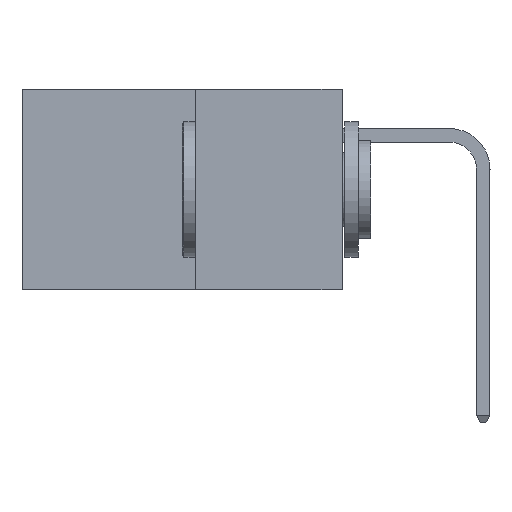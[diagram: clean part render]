
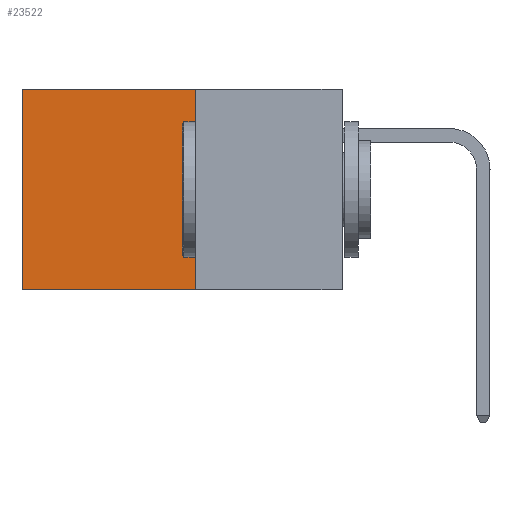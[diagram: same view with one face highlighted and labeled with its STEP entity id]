
A CAD part, left-side view. The second image highlights one B-rep face of the part: STEP entity #23522.
In plain terms, the highlighted planar face has unit normal (-1, 0, 0).
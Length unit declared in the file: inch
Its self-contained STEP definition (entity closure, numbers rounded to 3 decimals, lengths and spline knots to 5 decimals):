
#218 = ORIENTED_EDGE ( 'NONE', *, *, #18377, .T. ) ;
#535 = DIRECTION ( 'NONE',  ( 1., 0., 0. ) ) ;
#880 = LINE ( 'NONE', #8415, #6018 ) ;
#889 = EDGE_LOOP ( 'NONE', ( #14393, #20771, #14347, #218 ) ) ;
#1818 = LINE ( 'NONE', #4591, #18602 ) ;
#1972 = VERTEX_POINT ( 'NONE', #27036 ) ;
#4591 = CARTESIAN_POINT ( 'NONE',  ( 0.277, 0.59, -0.37 ) ) ;
#6018 = VECTOR ( 'NONE', #25820, 39.37008 ) ;
#6804 = DIRECTION ( 'NONE',  ( 0., 0., -1. ) ) ;
#6937 = VECTOR ( 'NONE', #21054, 39.37008 ) ;
#8415 = CARTESIAN_POINT ( 'NONE',  ( 0.277, 0.27, -0.37 ) ) ;
#9565 = DIRECTION ( 'NONE',  ( 0., 1., 0. ) ) ;
#9584 = LINE ( 'NONE', #26789, #14672 ) ;
#11181 = FACE_OUTER_BOUND ( 'NONE', #889, .T. ) ;
#12370 = CARTESIAN_POINT ( 'NONE',  ( 0.277, 0.27, -0.37 ) ) ;
#12713 = LINE ( 'NONE', #12370, #6937 ) ;
#13580 = VERTEX_POINT ( 'NONE', #25212 ) ;
#14347 = ORIENTED_EDGE ( 'NONE', *, *, #17163, .F. ) ;
#14393 = ORIENTED_EDGE ( 'NONE', *, *, #25401, .T. ) ;
#14672 = VECTOR ( 'NONE', #9565, 39.37008 ) ;
#15749 = CARTESIAN_POINT ( 'NONE',  ( 0.277, 0.27, -0.37 ) ) ;
#15768 = CARTESIAN_POINT ( 'NONE',  ( 0.277, 0.59, 0. ) ) ;
#15849 = DIRECTION ( 'NONE',  ( 0., 0., -1. ) ) ;
#15962 = VERTEX_POINT ( 'NONE', #26214 ) ;
#17163 = EDGE_CURVE ( 'NONE', #13580, #1972, #12713, .T. ) ;
#18377 = EDGE_CURVE ( 'NONE', #13580, #28013, #9584, .T. ) ;
#18602 = VECTOR ( 'NONE', #6804, 39.37008 ) ;
#19019 = AXIS2_PLACEMENT_3D ( 'NONE', #15749, #535, #15849 ) ;
#20771 = ORIENTED_EDGE ( 'NONE', *, *, #23920, .F. ) ;
#21054 = DIRECTION ( 'NONE',  ( 0., 0., -1. ) ) ;
#23522 = ADVANCED_FACE ( 'NONE', ( #11181 ), #26700, .F. ) ;
#23920 = EDGE_CURVE ( 'NONE', #1972, #15962, #880, .T. ) ;
#25212 = CARTESIAN_POINT ( 'NONE',  ( 0.277, 0.27, 0. ) ) ;
#25401 = EDGE_CURVE ( 'NONE', #28013, #15962, #1818, .T. ) ;
#25820 = DIRECTION ( 'NONE',  ( 0., 1., 0. ) ) ;
#26214 = CARTESIAN_POINT ( 'NONE',  ( 0.277, 0.59, -0.37 ) ) ;
#26700 = PLANE ( 'NONE',  #19019 ) ;
#26789 = CARTESIAN_POINT ( 'NONE',  ( 0.277, 0.27, 0. ) ) ;
#27036 = CARTESIAN_POINT ( 'NONE',  ( 0.277, 0.27, -0.37 ) ) ;
#28013 = VERTEX_POINT ( 'NONE', #15768 ) ;
